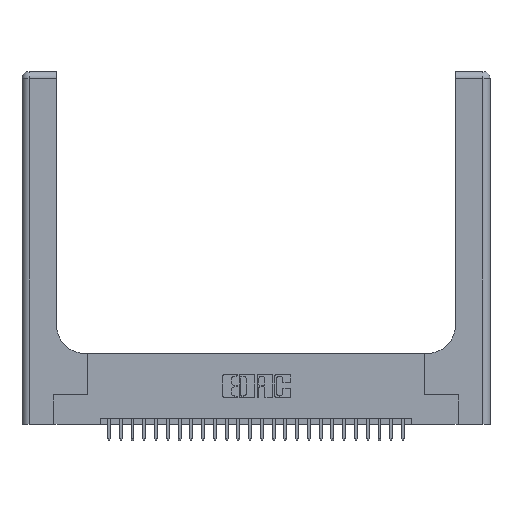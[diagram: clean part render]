
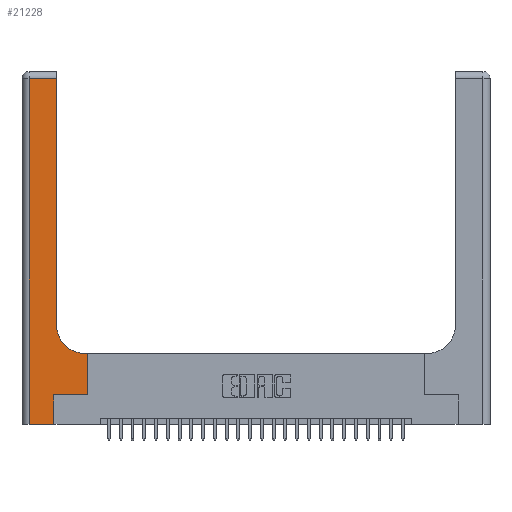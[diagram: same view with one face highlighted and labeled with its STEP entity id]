
A CAD part, top view. The second image highlights one B-rep face of the part: STEP entity #21228.
In plain terms, the highlighted planar face has unit normal (0, 0, 1).
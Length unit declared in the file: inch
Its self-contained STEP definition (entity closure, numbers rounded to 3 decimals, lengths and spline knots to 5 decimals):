
#426 = AXIS2_PLACEMENT_3D ( 'NONE', #20516, #14069, #1204 ) ;
#461 = DIRECTION ( 'NONE',  ( 1., 0., 0. ) ) ;
#507 = ORIENTED_EDGE ( 'NONE', *, *, #6557, .T. ) ;
#606 = VECTOR ( 'NONE', #4842, 39.37008 ) ;
#744 = CARTESIAN_POINT ( 'NONE',  ( 0.06, 0., 0.37 ) ) ;
#808 = LINE ( 'NONE', #11167, #25634 ) ;
#1204 = DIRECTION ( 'NONE',  ( -1., 0., 0. ) ) ;
#1374 = VERTEX_POINT ( 'NONE', #19488 ) ;
#1489 = CARTESIAN_POINT ( 'NONE',  ( 0.5585, 0.25, 0.37 ) ) ;
#1569 = VERTEX_POINT ( 'NONE', #14091 ) ;
#1852 = AXIS2_PLACEMENT_3D ( 'NONE', #4643, #8647, #2580 ) ;
#1930 = VERTEX_POINT ( 'NONE', #22916 ) ;
#2471 = VERTEX_POINT ( 'NONE', #744 ) ;
#2580 = DIRECTION ( 'NONE',  ( 1., 0., 0. ) ) ;
#2612 = VECTOR ( 'NONE', #4601, 39.37008 ) ;
#2873 = ORIENTED_EDGE ( 'NONE', *, *, #11910, .T. ) ;
#4129 = ORIENTED_EDGE ( 'NONE', *, *, #5149, .T. ) ;
#4601 = DIRECTION ( 'NONE',  ( -1., 0., 0. ) ) ;
#4643 = CARTESIAN_POINT ( 'NONE',  ( 0.5415, 0.85, 0.37 ) ) ;
#4798 = VECTOR ( 'NONE', #22055, 39.37008 ) ;
#4842 = DIRECTION ( 'NONE',  ( 1., 0., 0. ) ) ;
#5149 = EDGE_CURVE ( 'NONE', #22026, #1569, #19262, .T. ) ;
#5754 = LINE ( 'NONE', #5873, #20151 ) ;
#5873 = CARTESIAN_POINT ( 'NONE',  ( 0.269, 0., 0.37 ) ) ;
#6528 = VECTOR ( 'NONE', #20610, 39.37008 ) ;
#6557 = EDGE_CURVE ( 'NONE', #1374, #18266, #5754, .T. ) ;
#6702 = CARTESIAN_POINT ( 'NONE',  ( 0.2915, 3., 0.37 ) ) ;
#6839 = ORIENTED_EDGE ( 'NONE', *, *, #24411, .T. ) ;
#7307 = ORIENTED_EDGE ( 'NONE', *, *, #22207, .T. ) ;
#8268 = ORIENTED_EDGE ( 'NONE', *, *, #16912, .T. ) ;
#8647 = DIRECTION ( 'NONE',  ( 0., 0., -1. ) ) ;
#10318 = DIRECTION ( 'NONE',  ( 0., 1., 0. ) ) ;
#10339 = CIRCLE ( 'NONE', #1852, 0.25 ) ;
#10529 = VECTOR ( 'NONE', #27686, 39.37008 ) ;
#10574 = LINE ( 'NONE', #19690, #4798 ) ;
#10720 = ORIENTED_EDGE ( 'NONE', *, *, #22291, .T. ) ;
#11167 = CARTESIAN_POINT ( 'NONE',  ( 0., 0., 0.37 ) ) ;
#11910 = EDGE_CURVE ( 'NONE', #18266, #22026, #19738, .T. ) ;
#12083 = VERTEX_POINT ( 'NONE', #14094 ) ;
#12670 = VERTEX_POINT ( 'NONE', #13391 ) ;
#13391 = CARTESIAN_POINT ( 'NONE',  ( 0.2915, 2.94, 0.37 ) ) ;
#14069 = DIRECTION ( 'NONE',  ( 0., 0., -1. ) ) ;
#14091 = CARTESIAN_POINT ( 'NONE',  ( 0.5585, 0.6, 0.37 ) ) ;
#14094 = CARTESIAN_POINT ( 'NONE',  ( 0.06, 2.94, 0.37 ) ) ;
#14793 = CARTESIAN_POINT ( 'NONE',  ( 0.2915, 0.6, 0.37 ) ) ;
#15315 = CARTESIAN_POINT ( 'NONE',  ( 0., 2.94, 0.37 ) ) ;
#15758 = CARTESIAN_POINT ( 'NONE',  ( 0.269, 0.25, 0.37 ) ) ;
#16912 = EDGE_CURVE ( 'NONE', #1569, #18906, #25918, .T. ) ;
#17005 = FACE_OUTER_BOUND ( 'NONE', #20256, .T. ) ;
#17158 = LINE ( 'NONE', #6702, #25195 ) ;
#17762 = CARTESIAN_POINT ( 'NONE',  ( 0.5415, 0.6, 0.37 ) ) ;
#18266 = VERTEX_POINT ( 'NONE', #21198 ) ;
#18906 = VERTEX_POINT ( 'NONE', #17762 ) ;
#19040 = EDGE_CURVE ( 'NONE', #12670, #12083, #22463, .T. ) ;
#19262 = LINE ( 'NONE', #1489, #6528 ) ;
#19488 = CARTESIAN_POINT ( 'NONE',  ( 0.269, 0., 0.37 ) ) ;
#19690 = CARTESIAN_POINT ( 'NONE',  ( 0.06, 3., 0.37 ) ) ;
#19738 = LINE ( 'NONE', #15758, #606 ) ;
#20151 = VECTOR ( 'NONE', #10318, 39.37008 ) ;
#20256 = EDGE_LOOP ( 'NONE', ( #6839, #25072, #7307, #10720, #507, #2873, #4129, #8268, #26509 ) ) ;
#20516 = CARTESIAN_POINT ( 'NONE',  ( 0., 3., 0.37 ) ) ;
#20610 = DIRECTION ( 'NONE',  ( 0., 1., 0. ) ) ;
#21198 = CARTESIAN_POINT ( 'NONE',  ( 0.269, 0.25, 0.37 ) ) ;
#21228 = ADVANCED_FACE ( 'NONE', ( #17005 ), #26876, .F. ) ;
#22026 = VERTEX_POINT ( 'NONE', #23019 ) ;
#22055 = DIRECTION ( 'NONE',  ( 0., -1., 0. ) ) ;
#22207 = EDGE_CURVE ( 'NONE', #12083, #2471, #10574, .T. ) ;
#22291 = EDGE_CURVE ( 'NONE', #2471, #1374, #808, .T. ) ;
#22463 = LINE ( 'NONE', #15315, #2612 ) ;
#22916 = CARTESIAN_POINT ( 'NONE',  ( 0.2915, 0.85, 0.37 ) ) ;
#23019 = CARTESIAN_POINT ( 'NONE',  ( 0.5585, 0.25, 0.37 ) ) ;
#23673 = DIRECTION ( 'NONE',  ( 0., 1., 0. ) ) ;
#24411 = EDGE_CURVE ( 'NONE', #1930, #12670, #17158, .T. ) ;
#25072 = ORIENTED_EDGE ( 'NONE', *, *, #19040, .T. ) ;
#25195 = VECTOR ( 'NONE', #23673, 39.37008 ) ;
#25634 = VECTOR ( 'NONE', #461, 39.37008 ) ;
#25918 = LINE ( 'NONE', #14793, #10529 ) ;
#26241 = EDGE_CURVE ( 'NONE', #18906, #1930, #10339, .T. ) ;
#26509 = ORIENTED_EDGE ( 'NONE', *, *, #26241, .T. ) ;
#26876 = PLANE ( 'NONE',  #426 ) ;
#27686 = DIRECTION ( 'NONE',  ( -1., 0., 0. ) ) ;
